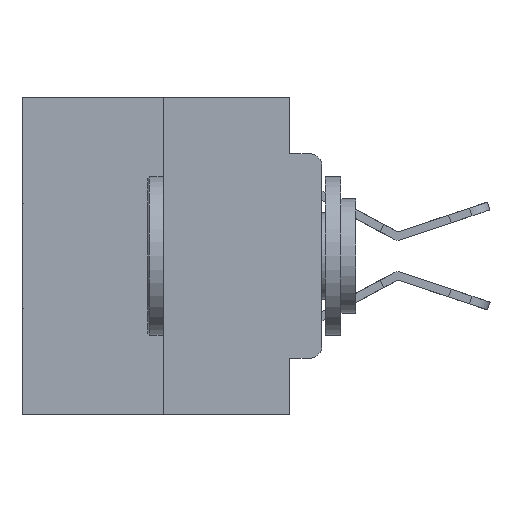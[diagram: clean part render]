
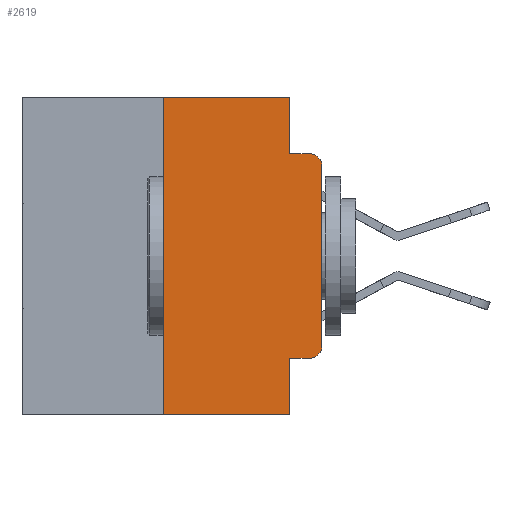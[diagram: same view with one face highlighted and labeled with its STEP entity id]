
A CAD part, left-side view. The second image highlights one B-rep face of the part: STEP entity #2619.
In plain terms, the highlighted planar face has unit normal (-1, 0, 0).
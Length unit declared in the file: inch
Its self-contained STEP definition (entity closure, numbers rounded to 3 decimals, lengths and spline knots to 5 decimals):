
#810 = DIRECTION ( 'NONE',  ( 0., 0., -1. ) ) ;
#1111 = ORIENTED_EDGE ( 'NONE', *, *, #23452, .F. ) ;
#1451 = VERTEX_POINT ( 'NONE', #24641 ) ;
#1958 = LINE ( 'NONE', #18070, #12365 ) ;
#2619 = ADVANCED_FACE ( 'NONE', ( #18690 ), #27898, .F. ) ;
#3638 = EDGE_CURVE ( 'NONE', #22622, #18617, #14555, .T. ) ;
#3744 = DIRECTION ( 'NONE',  ( 0., 0., -1. ) ) ;
#3861 = CARTESIAN_POINT ( 'NONE',  ( 0., 0.051, 0. ) ) ;
#3921 = CARTESIAN_POINT ( 'NONE',  ( 0., 0.02, -0.1085 ) ) ;
#4220 = VECTOR ( 'NONE', #27590, 39.37008 ) ;
#4569 = ORIENTED_EDGE ( 'NONE', *, *, #16167, .F. ) ;
#4841 = DIRECTION ( 'NONE',  ( 0., 0., -1. ) ) ;
#5224 = VERTEX_POINT ( 'NONE', #27355 ) ;
#6117 = CIRCLE ( 'NONE', #14785, 0.02 ) ;
#6151 = CARTESIAN_POINT ( 'NONE',  ( 0., 0.02, -0.3915 ) ) ;
#6831 = AXIS2_PLACEMENT_3D ( 'NONE', #3921, #11142, #8744 ) ;
#7254 = CARTESIAN_POINT ( 'NONE',  ( 0., 0.473, 0. ) ) ;
#7405 = DIRECTION ( 'NONE',  ( 0., -1., 0. ) ) ;
#7583 = LINE ( 'NONE', #19181, #29120 ) ;
#7832 = DIRECTION ( 'NONE',  ( -1., 0., 0. ) ) ;
#8140 = VECTOR ( 'NONE', #810, 39.37008 ) ;
#8744 = DIRECTION ( 'NONE',  ( 0., 0., -1. ) ) ;
#8996 = AXIS2_PLACEMENT_3D ( 'NONE', #7254, #16426, #25620 ) ;
#9725 = VERTEX_POINT ( 'NONE', #13714 ) ;
#9943 = EDGE_CURVE ( 'NONE', #27489, #5224, #6117, .T. ) ;
#10210 = ORIENTED_EDGE ( 'NONE', *, *, #28244, .F. ) ;
#10396 = VECTOR ( 'NONE', #25418, 39.37008 ) ;
#10814 = EDGE_CURVE ( 'NONE', #23586, #22622, #13418, .T. ) ;
#11142 = DIRECTION ( 'NONE',  ( -1., 0., 0. ) ) ;
#11252 = LINE ( 'NONE', #20896, #10396 ) ;
#12282 = CARTESIAN_POINT ( 'NONE',  ( 0., 0.473, 0. ) ) ;
#12365 = VECTOR ( 'NONE', #18220, 39.37008 ) ;
#12779 = VERTEX_POINT ( 'NONE', #29045 ) ;
#12975 = VERTEX_POINT ( 'NONE', #17876 ) ;
#13196 = ORIENTED_EDGE ( 'NONE', *, *, #26122, .T. ) ;
#13350 = ORIENTED_EDGE ( 'NONE', *, *, #3638, .F. ) ;
#13418 = LINE ( 'NONE', #25328, #4220 ) ;
#13714 = CARTESIAN_POINT ( 'NONE',  ( 0., 0., -0.1085 ) ) ;
#14363 = ORIENTED_EDGE ( 'NONE', *, *, #9943, .T. ) ;
#14517 = DIRECTION ( 'NONE',  ( 0., 0., 1. ) ) ;
#14555 = LINE ( 'NONE', #12282, #15603 ) ;
#14702 = CARTESIAN_POINT ( 'NONE',  ( 0., 0.25, -0.5 ) ) ;
#14785 = AXIS2_PLACEMENT_3D ( 'NONE', #6151, #7832, #3744 ) ;
#15603 = VECTOR ( 'NONE', #21481, 39.37008 ) ;
#16009 = CARTESIAN_POINT ( 'NONE',  ( 0., 0.25, 0. ) ) ;
#16167 = EDGE_CURVE ( 'NONE', #1451, #12779, #18407, .T. ) ;
#16212 = EDGE_CURVE ( 'NONE', #1451, #27489, #20971, .T. ) ;
#16426 = DIRECTION ( 'NONE',  ( 1., 0., 0. ) ) ;
#16519 = EDGE_CURVE ( 'NONE', #9725, #17665, #28974, .T. ) ;
#17665 = VERTEX_POINT ( 'NONE', #17968 ) ;
#17876 = CARTESIAN_POINT ( 'NONE',  ( 0., 0.051, -0.0885 ) ) ;
#17968 = CARTESIAN_POINT ( 'NONE',  ( 0., 0.02, -0.0885 ) ) ;
#18070 = CARTESIAN_POINT ( 'NONE',  ( 0., 0.473, -0.5 ) ) ;
#18220 = DIRECTION ( 'NONE',  ( 0., -1., 0. ) ) ;
#18407 = LINE ( 'NONE', #27613, #23185 ) ;
#18617 = VERTEX_POINT ( 'NONE', #3861 ) ;
#18690 = FACE_OUTER_BOUND ( 'NONE', #24643, .T. ) ;
#19181 = CARTESIAN_POINT ( 'NONE',  ( 0., 0., 0. ) ) ;
#20896 = CARTESIAN_POINT ( 'NONE',  ( 0., 0.051, -0.0885 ) ) ;
#20971 = LINE ( 'NONE', #23095, #28007 ) ;
#21214 = ORIENTED_EDGE ( 'NONE', *, *, #10814, .F. ) ;
#21481 = DIRECTION ( 'NONE',  ( 0., -1., 0. ) ) ;
#22622 = VERTEX_POINT ( 'NONE', #16009 ) ;
#22717 = EDGE_CURVE ( 'NONE', #5224, #9725, #7583, .T. ) ;
#23095 = CARTESIAN_POINT ( 'NONE',  ( 0., 0.051, -0.4115 ) ) ;
#23185 = VECTOR ( 'NONE', #4841, 39.37008 ) ;
#23452 = EDGE_CURVE ( 'NONE', #12975, #17665, #11252, .T. ) ;
#23586 = VERTEX_POINT ( 'NONE', #14702 ) ;
#24397 = CARTESIAN_POINT ( 'NONE',  ( 0., 0.02, -0.4115 ) ) ;
#24641 = CARTESIAN_POINT ( 'NONE',  ( 0., 0.051, -0.4115 ) ) ;
#24643 = EDGE_LOOP ( 'NONE', ( #29602, #25876, #1111, #10210, #13350, #21214, #13196, #4569, #25676, #14363 ) ) ;
#25328 = CARTESIAN_POINT ( 'NONE',  ( 0., 0.25, 0. ) ) ;
#25418 = DIRECTION ( 'NONE',  ( 0., -1., 0. ) ) ;
#25620 = DIRECTION ( 'NONE',  ( 0., 0., -1. ) ) ;
#25676 = ORIENTED_EDGE ( 'NONE', *, *, #16212, .T. ) ;
#25876 = ORIENTED_EDGE ( 'NONE', *, *, #16519, .T. ) ;
#26122 = EDGE_CURVE ( 'NONE', #23586, #12779, #1958, .T. ) ;
#26728 = LINE ( 'NONE', #28700, #8140 ) ;
#27355 = CARTESIAN_POINT ( 'NONE',  ( 0., 0., -0.3915 ) ) ;
#27489 = VERTEX_POINT ( 'NONE', #24397 ) ;
#27590 = DIRECTION ( 'NONE',  ( 0., 0., 1. ) ) ;
#27613 = CARTESIAN_POINT ( 'NONE',  ( 0., 0.051, 0. ) ) ;
#27898 = PLANE ( 'NONE',  #8996 ) ;
#28007 = VECTOR ( 'NONE', #7405, 39.37008 ) ;
#28244 = EDGE_CURVE ( 'NONE', #18617, #12975, #26728, .T. ) ;
#28700 = CARTESIAN_POINT ( 'NONE',  ( 0., 0.051, 0. ) ) ;
#28974 = CIRCLE ( 'NONE', #6831, 0.02 ) ;
#29045 = CARTESIAN_POINT ( 'NONE',  ( 0., 0.051, -0.5 ) ) ;
#29120 = VECTOR ( 'NONE', #14517, 39.37008 ) ;
#29602 = ORIENTED_EDGE ( 'NONE', *, *, #22717, .T. ) ;
